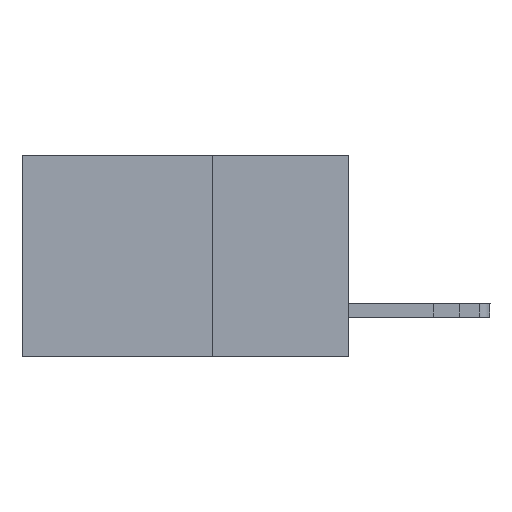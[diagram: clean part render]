
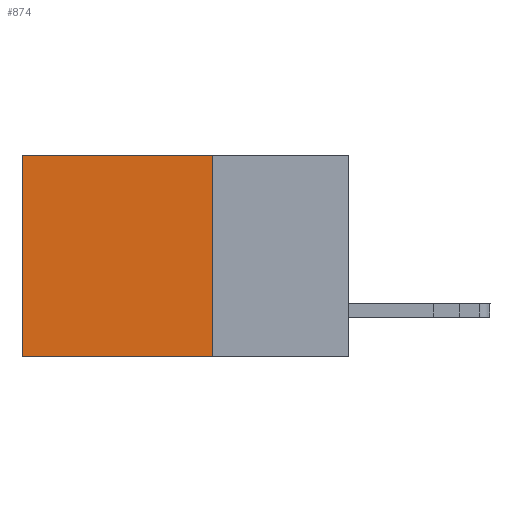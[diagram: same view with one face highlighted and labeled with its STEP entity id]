
A CAD part, left-side view. The second image highlights one B-rep face of the part: STEP entity #874.
In plain terms, the highlighted planar face has unit normal (-1, 0, 0).
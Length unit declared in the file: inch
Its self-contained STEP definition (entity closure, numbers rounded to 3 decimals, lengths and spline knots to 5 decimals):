
#374 = LINE ( 'NONE', #16611, #10576 ) ;
#874 = ADVANCED_FACE ( 'NONE', ( #4344 ), #4530, .F. ) ;
#875 = CARTESIAN_POINT ( 'NONE',  ( 0.298, 0.25, -0.37 ) ) ;
#2697 = DIRECTION ( 'NONE',  ( 0., 0., -1. ) ) ;
#3116 = DIRECTION ( 'NONE',  ( 0., 0., -1. ) ) ;
#3337 = DIRECTION ( 'NONE',  ( 0., 1., 0. ) ) ;
#3672 = LINE ( 'NONE', #10249, #8218 ) ;
#4112 = ORIENTED_EDGE ( 'NONE', *, *, #4478, .T. ) ;
#4170 = DIRECTION ( 'NONE',  ( 1., 0., 0. ) ) ;
#4344 = FACE_OUTER_BOUND ( 'NONE', #10669, .T. ) ;
#4478 = EDGE_CURVE ( 'NONE', #17604, #5410, #374, .T. ) ;
#4530 = PLANE ( 'NONE',  #18828 ) ;
#5410 = VERTEX_POINT ( 'NONE', #8273 ) ;
#6113 = VERTEX_POINT ( 'NONE', #11727 ) ;
#8218 = VECTOR ( 'NONE', #16108, 39.37008 ) ;
#8273 = CARTESIAN_POINT ( 'NONE',  ( 0.298, 0.6, 0. ) ) ;
#8424 = CARTESIAN_POINT ( 'NONE',  ( 0.298, 0.25, 0. ) ) ;
#9596 = VECTOR ( 'NONE', #10608, 39.37008 ) ;
#10098 = CARTESIAN_POINT ( 'NONE',  ( 0.298, 0.25, 0. ) ) ;
#10249 = CARTESIAN_POINT ( 'NONE',  ( 0.298, 0.6, 0. ) ) ;
#10334 = CARTESIAN_POINT ( 'NONE',  ( 0.298, 0.25, 0. ) ) ;
#10576 = VECTOR ( 'NONE', #3337, 39.37008 ) ;
#10608 = DIRECTION ( 'NONE',  ( 0., 1., 0. ) ) ;
#10669 = EDGE_LOOP ( 'NONE', ( #17072, #15745, #18882, #4112 ) ) ;
#11304 = VERTEX_POINT ( 'NONE', #11988 ) ;
#11727 = CARTESIAN_POINT ( 'NONE',  ( 0.298, 0.6, -0.37 ) ) ;
#11988 = CARTESIAN_POINT ( 'NONE',  ( 0.298, 0.25, -0.37 ) ) ;
#12140 = LINE ( 'NONE', #875, #9596 ) ;
#12154 = EDGE_CURVE ( 'NONE', #17604, #11304, #15781, .T. ) ;
#13493 = EDGE_CURVE ( 'NONE', #11304, #6113, #12140, .T. ) ;
#15745 = ORIENTED_EDGE ( 'NONE', *, *, #13493, .F. ) ;
#15781 = LINE ( 'NONE', #10098, #18412 ) ;
#16080 = EDGE_CURVE ( 'NONE', #5410, #6113, #3672, .T. ) ;
#16108 = DIRECTION ( 'NONE',  ( 0., 0., -1. ) ) ;
#16611 = CARTESIAN_POINT ( 'NONE',  ( 0.298, 0.25, 0. ) ) ;
#17072 = ORIENTED_EDGE ( 'NONE', *, *, #16080, .T. ) ;
#17604 = VERTEX_POINT ( 'NONE', #8424 ) ;
#18412 = VECTOR ( 'NONE', #2697, 39.37008 ) ;
#18828 = AXIS2_PLACEMENT_3D ( 'NONE', #10334, #4170, #3116 ) ;
#18882 = ORIENTED_EDGE ( 'NONE', *, *, #12154, .F. ) ;
